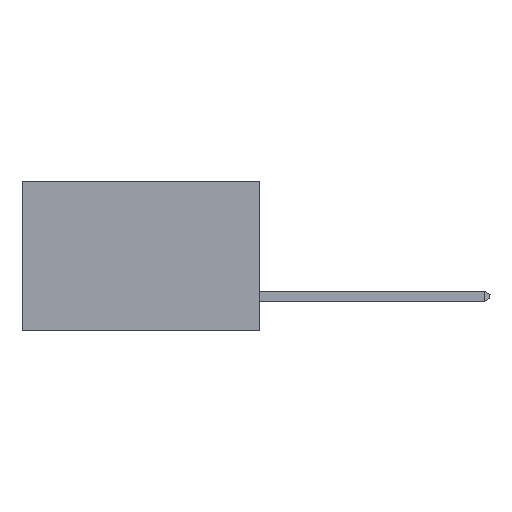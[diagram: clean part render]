
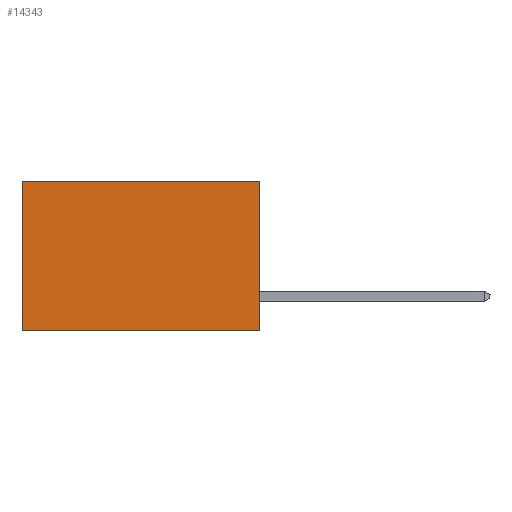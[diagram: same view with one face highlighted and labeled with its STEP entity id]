
A CAD part, left-side view. The second image highlights one B-rep face of the part: STEP entity #14343.
In plain terms, the highlighted planar face has unit normal (-1, 0, 0).
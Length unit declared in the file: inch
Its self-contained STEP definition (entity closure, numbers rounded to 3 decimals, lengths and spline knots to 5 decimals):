
#80 = FACE_OUTER_BOUND ( 'NONE', #386, .T. ) ;
#386 = EDGE_LOOP ( 'NONE', ( #22848, #4936, #13357, #21481 ) ) ;
#1654 = VECTOR ( 'NONE', #17690, 39.37008 ) ;
#1762 = VECTOR ( 'NONE', #17964, 39.37008 ) ;
#1820 = VERTEX_POINT ( 'NONE', #10934 ) ;
#2360 = LINE ( 'NONE', #2486, #1762 ) ;
#2486 = CARTESIAN_POINT ( 'NONE',  ( 0.277, 0.59, -0.37 ) ) ;
#2499 = CARTESIAN_POINT ( 'NONE',  ( 0.277, 0., -0.37 ) ) ;
#4936 = ORIENTED_EDGE ( 'NONE', *, *, #15794, .F. ) ;
#5390 = CARTESIAN_POINT ( 'NONE',  ( 0.277, 0.59, 0. ) ) ;
#6733 = EDGE_CURVE ( 'NONE', #21384, #21697, #9417, .T. ) ;
#7499 = CARTESIAN_POINT ( 'NONE',  ( 0.277, 0., 0. ) ) ;
#7519 = DIRECTION ( 'NONE',  ( 0., 1., 0. ) ) ;
#8159 = CARTESIAN_POINT ( 'NONE',  ( 0.277, 0., 0. ) ) ;
#8318 = DIRECTION ( 'NONE',  ( 1., 0., 0. ) ) ;
#9003 = EDGE_CURVE ( 'NONE', #21697, #1820, #2360, .T. ) ;
#9417 = LINE ( 'NONE', #7499, #24038 ) ;
#10934 = CARTESIAN_POINT ( 'NONE',  ( 0.277, 0.59, -0.37 ) ) ;
#11929 = LINE ( 'NONE', #21476, #1654 ) ;
#13357 = ORIENTED_EDGE ( 'NONE', *, *, #14498, .F. ) ;
#14343 = ADVANCED_FACE ( 'NONE', ( #80 ), #19872, .F. ) ;
#14498 = EDGE_CURVE ( 'NONE', #21384, #15858, #11929, .T. ) ;
#15517 = CARTESIAN_POINT ( 'NONE',  ( 0.277, 0., -0.37 ) ) ;
#15794 = EDGE_CURVE ( 'NONE', #15858, #1820, #20877, .T. ) ;
#15858 = VERTEX_POINT ( 'NONE', #17634 ) ;
#16712 = AXIS2_PLACEMENT_3D ( 'NONE', #2499, #8318, #21759 ) ;
#17459 = DIRECTION ( 'NONE',  ( 0., 1., 0. ) ) ;
#17634 = CARTESIAN_POINT ( 'NONE',  ( 0.277, 0., -0.37 ) ) ;
#17690 = DIRECTION ( 'NONE',  ( 0., 0., -1. ) ) ;
#17964 = DIRECTION ( 'NONE',  ( 0., 0., -1. ) ) ;
#19872 = PLANE ( 'NONE',  #16712 ) ;
#20291 = VECTOR ( 'NONE', #17459, 39.37008 ) ;
#20877 = LINE ( 'NONE', #15517, #20291 ) ;
#21384 = VERTEX_POINT ( 'NONE', #8159 ) ;
#21476 = CARTESIAN_POINT ( 'NONE',  ( 0.277, 0., -0.37 ) ) ;
#21481 = ORIENTED_EDGE ( 'NONE', *, *, #6733, .T. ) ;
#21697 = VERTEX_POINT ( 'NONE', #5390 ) ;
#21759 = DIRECTION ( 'NONE',  ( 0., 0., -1. ) ) ;
#22848 = ORIENTED_EDGE ( 'NONE', *, *, #9003, .T. ) ;
#24038 = VECTOR ( 'NONE', #7519, 39.37008 ) ;
